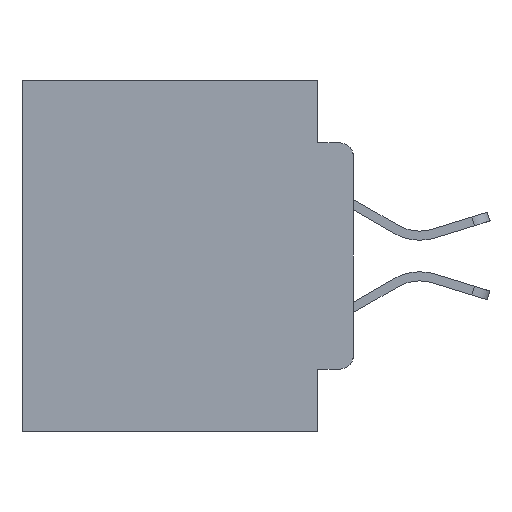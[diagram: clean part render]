
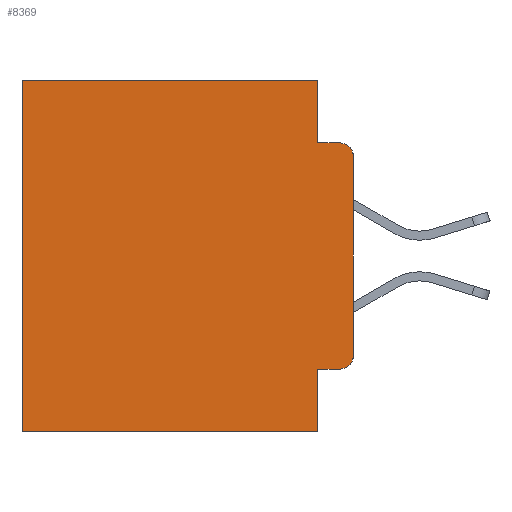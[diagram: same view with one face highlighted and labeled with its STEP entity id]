
A CAD part, left-side view. The second image highlights one B-rep face of the part: STEP entity #8369.
In plain terms, the highlighted planar face has unit normal (-1, 0, 0).
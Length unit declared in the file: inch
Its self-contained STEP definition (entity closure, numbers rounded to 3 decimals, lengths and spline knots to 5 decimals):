
#176 = VECTOR ( 'NONE', #5768, 39.37008 ) ;
#786 = VERTEX_POINT ( 'NONE', #23665 ) ;
#1002 = CARTESIAN_POINT ( 'NONE',  ( 0.298, 0.02, -0.3915 ) ) ;
#1316 = EDGE_CURVE ( 'NONE', #5258, #13267, #21822, .T. ) ;
#1759 = CARTESIAN_POINT ( 'NONE',  ( 0.298, 0.051, -0.4115 ) ) ;
#2143 = CARTESIAN_POINT ( 'NONE',  ( 0.298, 0.473, 0. ) ) ;
#2205 = VERTEX_POINT ( 'NONE', #15949 ) ;
#2712 = DIRECTION ( 'NONE',  ( 0., 0., -1. ) ) ;
#2720 = DIRECTION ( 'NONE',  ( 0., 1., 0. ) ) ;
#3355 = ORIENTED_EDGE ( 'NONE', *, *, #27264, .T. ) ;
#3380 = AXIS2_PLACEMENT_3D ( 'NONE', #11185, #9364, #2712 ) ;
#3388 = DIRECTION ( 'NONE',  ( 0., 0., -1. ) ) ;
#3800 = LINE ( 'NONE', #6056, #26899 ) ;
#4199 = PLANE ( 'NONE',  #24164 ) ;
#4611 = DIRECTION ( 'NONE',  ( 0., 0., -1. ) ) ;
#5258 = VERTEX_POINT ( 'NONE', #13789 ) ;
#5768 = DIRECTION ( 'NONE',  ( 0., 0., -1. ) ) ;
#6056 = CARTESIAN_POINT ( 'NONE',  ( 0.298, 0.051, 0. ) ) ;
#6329 = CARTESIAN_POINT ( 'NONE',  ( 0.298, 0., -0.3915 ) ) ;
#6547 = DIRECTION ( 'NONE',  ( 0., 0., -1. ) ) ;
#7719 = VECTOR ( 'NONE', #4611, 39.37008 ) ;
#7757 = DIRECTION ( 'NONE',  ( 0., 1., 0. ) ) ;
#8369 = ADVANCED_FACE ( 'NONE', ( #23037 ), #4199, .F. ) ;
#8841 = ORIENTED_EDGE ( 'NONE', *, *, #22053, .F. ) ;
#9364 = DIRECTION ( 'NONE',  ( -1., 0., 0. ) ) ;
#10881 = ORIENTED_EDGE ( 'NONE', *, *, #17172, .T. ) ;
#10930 = ORIENTED_EDGE ( 'NONE', *, *, #1316, .T. ) ;
#10976 = CARTESIAN_POINT ( 'NONE',  ( 0.298, 0., 0. ) ) ;
#11185 = CARTESIAN_POINT ( 'NONE',  ( 0.298, 0.02, -0.1085 ) ) ;
#11359 = EDGE_CURVE ( 'NONE', #23203, #17502, #16941, .T. ) ;
#11447 = CARTESIAN_POINT ( 'NONE',  ( 0.298, 0.051, -0.0885 ) ) ;
#11509 = VERTEX_POINT ( 'NONE', #22786 ) ;
#11838 = CARTESIAN_POINT ( 'NONE',  ( 0.298, 0.02, -0.4115 ) ) ;
#12642 = ORIENTED_EDGE ( 'NONE', *, *, #25971, .F. ) ;
#12985 = VECTOR ( 'NONE', #7757, 39.37008 ) ;
#13194 = VERTEX_POINT ( 'NONE', #6329 ) ;
#13267 = VERTEX_POINT ( 'NONE', #22227 ) ;
#13446 = CARTESIAN_POINT ( 'NONE',  ( 0.298, 0.051, 0. ) ) ;
#13789 = CARTESIAN_POINT ( 'NONE',  ( 0.298, 0., -0.1085 ) ) ;
#14420 = VERTEX_POINT ( 'NONE', #1759 ) ;
#14481 = DIRECTION ( 'NONE',  ( 0., -1., 0. ) ) ;
#15046 = ORIENTED_EDGE ( 'NONE', *, *, #21285, .F. ) ;
#15897 = EDGE_LOOP ( 'NONE', ( #12642, #10930, #8841, #23410, #3355, #16104, #26506, #15046, #28137, #10881 ) ) ;
#15949 = CARTESIAN_POINT ( 'NONE',  ( 0.298, 0.473, 0. ) ) ;
#16104 = ORIENTED_EDGE ( 'NONE', *, *, #27638, .T. ) ;
#16254 = CARTESIAN_POINT ( 'NONE',  ( 0.298, 0., -0.5 ) ) ;
#16255 = VECTOR ( 'NONE', #22316, 39.37008 ) ;
#16729 = VECTOR ( 'NONE', #2720, 39.37008 ) ;
#16882 = DIRECTION ( 'NONE',  ( -1., 0., 0. ) ) ;
#16941 = LINE ( 'NONE', #13446, #16255 ) ;
#17172 = EDGE_CURVE ( 'NONE', #22280, #13194, #22814, .T. ) ;
#17502 = VERTEX_POINT ( 'NONE', #11447 ) ;
#18361 = LINE ( 'NONE', #21428, #176 ) ;
#19953 = DIRECTION ( 'NONE',  ( 1., 0., 0. ) ) ;
#19977 = LINE ( 'NONE', #22353, #25111 ) ;
#21180 = EDGE_CURVE ( 'NONE', #14420, #22280, #24474, .T. ) ;
#21275 = LINE ( 'NONE', #16254, #16729 ) ;
#21285 = EDGE_CURVE ( 'NONE', #14420, #786, #3800, .T. ) ;
#21428 = CARTESIAN_POINT ( 'NONE',  ( 0.298, 0., 0. ) ) ;
#21711 = DIRECTION ( 'NONE',  ( 0., 0., -1. ) ) ;
#21822 = CIRCLE ( 'NONE', #3380, 0.02 ) ;
#22053 = EDGE_CURVE ( 'NONE', #17502, #13267, #19977, .T. ) ;
#22227 = CARTESIAN_POINT ( 'NONE',  ( 0.298, 0.02, -0.0885 ) ) ;
#22280 = VERTEX_POINT ( 'NONE', #11838 ) ;
#22316 = DIRECTION ( 'NONE',  ( 0., 0., -1. ) ) ;
#22353 = CARTESIAN_POINT ( 'NONE',  ( 0.298, 0.051, -0.0885 ) ) ;
#22786 = CARTESIAN_POINT ( 'NONE',  ( 0.298, 0.473, -0.5 ) ) ;
#22814 = CIRCLE ( 'NONE', #27796, 0.02 ) ;
#22880 = EDGE_CURVE ( 'NONE', #786, #11509, #21275, .T. ) ;
#23037 = FACE_OUTER_BOUND ( 'NONE', #15897, .T. ) ;
#23203 = VERTEX_POINT ( 'NONE', #28293 ) ;
#23332 = CARTESIAN_POINT ( 'NONE',  ( 0.298, 0., 0. ) ) ;
#23410 = ORIENTED_EDGE ( 'NONE', *, *, #11359, .F. ) ;
#23446 = CARTESIAN_POINT ( 'NONE',  ( 0.298, 0.051, -0.4115 ) ) ;
#23665 = CARTESIAN_POINT ( 'NONE',  ( 0.298, 0.051, -0.5 ) ) ;
#23798 = VECTOR ( 'NONE', #14481, 39.37008 ) ;
#24164 = AXIS2_PLACEMENT_3D ( 'NONE', #10976, #19953, #6547 ) ;
#24474 = LINE ( 'NONE', #23446, #23798 ) ;
#24796 = LINE ( 'NONE', #23332, #12985 ) ;
#25111 = VECTOR ( 'NONE', #26794, 39.37008 ) ;
#25971 = EDGE_CURVE ( 'NONE', #5258, #13194, #18361, .T. ) ;
#26169 = LINE ( 'NONE', #2143, #7719 ) ;
#26506 = ORIENTED_EDGE ( 'NONE', *, *, #22880, .F. ) ;
#26794 = DIRECTION ( 'NONE',  ( 0., -1., 0. ) ) ;
#26899 = VECTOR ( 'NONE', #21711, 39.37008 ) ;
#27264 = EDGE_CURVE ( 'NONE', #23203, #2205, #24796, .T. ) ;
#27638 = EDGE_CURVE ( 'NONE', #2205, #11509, #26169, .T. ) ;
#27796 = AXIS2_PLACEMENT_3D ( 'NONE', #1002, #16882, #3388 ) ;
#28137 = ORIENTED_EDGE ( 'NONE', *, *, #21180, .T. ) ;
#28293 = CARTESIAN_POINT ( 'NONE',  ( 0.298, 0.051, 0. ) ) ;
